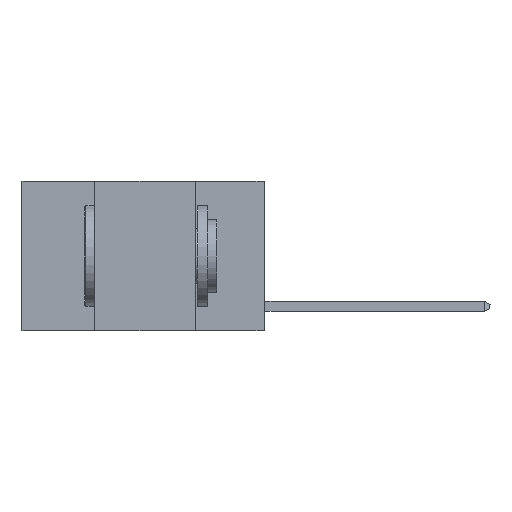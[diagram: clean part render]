
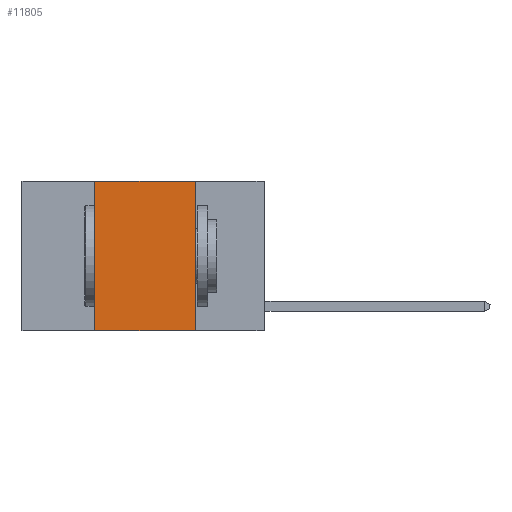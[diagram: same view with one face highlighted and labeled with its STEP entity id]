
A CAD part, left-side view. The second image highlights one B-rep face of the part: STEP entity #11805.
In plain terms, the highlighted planar face has unit normal (-1, 0, 0).
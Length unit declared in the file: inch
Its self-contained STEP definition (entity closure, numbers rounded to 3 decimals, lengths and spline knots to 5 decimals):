
#104 = CARTESIAN_POINT ( 'NONE',  ( 0., 0.17, 0. ) ) ;
#338 = AXIS2_PLACEMENT_3D ( 'NONE', #1831, #5875, #7071 ) ;
#1122 = CARTESIAN_POINT ( 'NONE',  ( 0., 0.42, 0. ) ) ;
#1181 = DIRECTION ( 'NONE',  ( 0., 0., -1. ) ) ;
#1831 = CARTESIAN_POINT ( 'NONE',  ( 0., 0.6, 0. ) ) ;
#2069 = CARTESIAN_POINT ( 'NONE',  ( 0., 0.42, 0. ) ) ;
#2238 = FACE_OUTER_BOUND ( 'NONE', #13499, .T. ) ;
#2790 = VERTEX_POINT ( 'NONE', #2069 ) ;
#2880 = ORIENTED_EDGE ( 'NONE', *, *, #7821, .F. ) ;
#3084 = VECTOR ( 'NONE', #10628, 39.37008 ) ;
#3097 = LINE ( 'NONE', #104, #10249 ) ;
#3917 = EDGE_CURVE ( 'NONE', #5076, #2790, #9101, .T. ) ;
#4537 = EDGE_CURVE ( 'NONE', #5076, #9620, #10846, .T. ) ;
#5076 = VERTEX_POINT ( 'NONE', #8571 ) ;
#5859 = CARTESIAN_POINT ( 'NONE',  ( 0., 0.6, 0. ) ) ;
#5875 = DIRECTION ( 'NONE',  ( 1., 0., 0. ) ) ;
#6537 = ORIENTED_EDGE ( 'NONE', *, *, #3917, .F. ) ;
#7071 = DIRECTION ( 'NONE',  ( 0., 0., -1. ) ) ;
#7821 = EDGE_CURVE ( 'NONE', #2790, #8625, #9857, .T. ) ;
#8571 = CARTESIAN_POINT ( 'NONE',  ( 0., 0.42, -0.37 ) ) ;
#8625 = VERTEX_POINT ( 'NONE', #9872 ) ;
#9101 = LINE ( 'NONE', #1122, #3084 ) ;
#9293 = PLANE ( 'NONE',  #338 ) ;
#9620 = VERTEX_POINT ( 'NONE', #10389 ) ;
#9857 = LINE ( 'NONE', #5859, #12819 ) ;
#9872 = CARTESIAN_POINT ( 'NONE',  ( 0., 0.17, 0. ) ) ;
#10249 = VECTOR ( 'NONE', #1181, 39.37008 ) ;
#10389 = CARTESIAN_POINT ( 'NONE',  ( 0., 0.17, -0.37 ) ) ;
#10628 = DIRECTION ( 'NONE',  ( 0., 0., 1. ) ) ;
#10812 = EDGE_CURVE ( 'NONE', #8625, #9620, #3097, .T. ) ;
#10846 = LINE ( 'NONE', #13657, #13519 ) ;
#11431 = DIRECTION ( 'NONE',  ( 0., -1., 0. ) ) ;
#11805 = ADVANCED_FACE ( 'NONE', ( #2238 ), #9293, .F. ) ;
#12638 = ORIENTED_EDGE ( 'NONE', *, *, #10812, .F. ) ;
#12819 = VECTOR ( 'NONE', #13271, 39.37008 ) ;
#13271 = DIRECTION ( 'NONE',  ( 0., -1., 0. ) ) ;
#13363 = ORIENTED_EDGE ( 'NONE', *, *, #4537, .T. ) ;
#13499 = EDGE_LOOP ( 'NONE', ( #12638, #2880, #6537, #13363 ) ) ;
#13519 = VECTOR ( 'NONE', #11431, 39.37008 ) ;
#13657 = CARTESIAN_POINT ( 'NONE',  ( 0., 0.6, -0.37 ) ) ;
